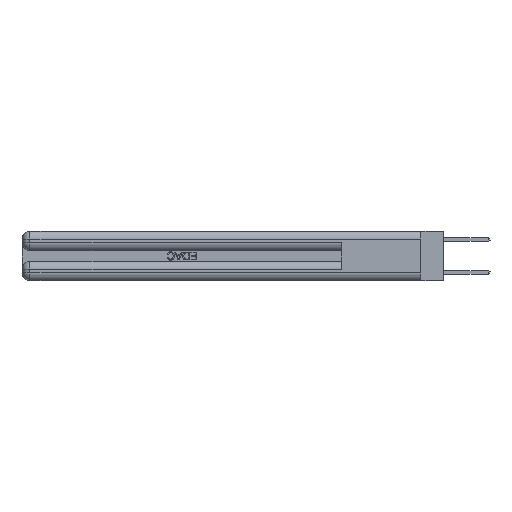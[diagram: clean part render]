
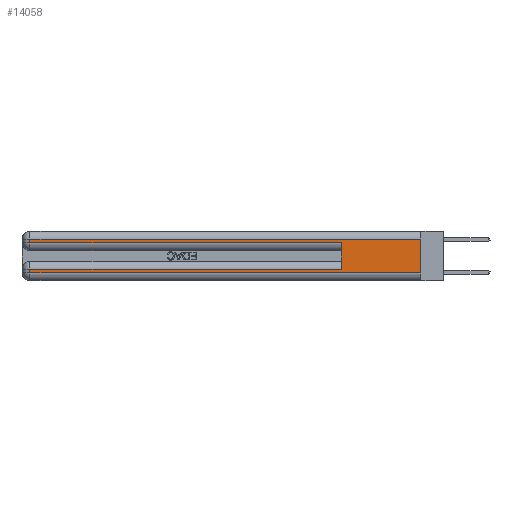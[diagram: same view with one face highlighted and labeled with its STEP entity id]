
A CAD part, left-side view. The second image highlights one B-rep face of the part: STEP entity #14058.
In plain terms, the highlighted planar face has unit normal (-1, 0, 0).
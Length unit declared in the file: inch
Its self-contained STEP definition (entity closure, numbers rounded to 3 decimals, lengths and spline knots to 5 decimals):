
#309 = VECTOR ( 'NONE', #28765, 39.37008 ) ;
#1189 = EDGE_CURVE ( 'NONE', #12646, #17756, #11935, .T. ) ;
#1290 = VECTOR ( 'NONE', #28421, 39.37008 ) ;
#1378 = LINE ( 'NONE', #26140, #14333 ) ;
#1954 = CARTESIAN_POINT ( 'NONE',  ( 0., 0., 0.06 ) ) ;
#2034 = DIRECTION ( 'NONE',  ( 0., 1., 0. ) ) ;
#3060 = DIRECTION ( 'NONE',  ( 0., 0., -1. ) ) ;
#3220 = VERTEX_POINT ( 'NONE', #25438 ) ;
#4101 = ORIENTED_EDGE ( 'NONE', *, *, #23650, .T. ) ;
#4545 = DIRECTION ( 'NONE',  ( 0., -1., 0. ) ) ;
#4770 = VECTOR ( 'NONE', #29475, 39.37008 ) ;
#5041 = VECTOR ( 'NONE', #29086, 39.37008 ) ;
#5283 = EDGE_LOOP ( 'NONE', ( #7089, #4101, #10918, #25118, #6736, #8065, #23968, #16320 ) ) ;
#6498 = LINE ( 'NONE', #11570, #12587 ) ;
#6736 = ORIENTED_EDGE ( 'NONE', *, *, #1189, .F. ) ;
#7089 = ORIENTED_EDGE ( 'NONE', *, *, #25392, .F. ) ;
#8065 = ORIENTED_EDGE ( 'NONE', *, *, #8126, .T. ) ;
#8126 = EDGE_CURVE ( 'NONE', #12646, #19858, #32157, .T. ) ;
#8192 = CARTESIAN_POINT ( 'NONE',  ( 0., 2.94, 0.37 ) ) ;
#8546 = AXIS2_PLACEMENT_3D ( 'NONE', #15978, #18500, #3060 ) ;
#10476 = CARTESIAN_POINT ( 'NONE',  ( 0., 0., 0.31 ) ) ;
#10918 = ORIENTED_EDGE ( 'NONE', *, *, #13367, .T. ) ;
#11570 = CARTESIAN_POINT ( 'NONE',  ( 0., 0., 0.37 ) ) ;
#11935 = LINE ( 'NONE', #18733, #5041 ) ;
#12197 = CARTESIAN_POINT ( 'NONE',  ( 0., 2.94, 0.06 ) ) ;
#12587 = VECTOR ( 'NONE', #20581, 39.37008 ) ;
#12646 = VERTEX_POINT ( 'NONE', #30498 ) ;
#12924 = EDGE_CURVE ( 'NONE', #19858, #27780, #31333, .T. ) ;
#13351 = VECTOR ( 'NONE', #2034, 39.37008 ) ;
#13367 = EDGE_CURVE ( 'NONE', #3220, #16617, #27677, .T. ) ;
#13630 = FACE_OUTER_BOUND ( 'NONE', #5283, .T. ) ;
#14058 = ADVANCED_FACE ( 'NONE', ( #13630 ), #31313, .F. ) ;
#14333 = VECTOR ( 'NONE', #31314, 39.37008 ) ;
#14904 = VECTOR ( 'NONE', #4545, 39.37008 ) ;
#15214 = VERTEX_POINT ( 'NONE', #23761 ) ;
#15978 = CARTESIAN_POINT ( 'NONE',  ( 0., 0., 0.37 ) ) ;
#16320 = ORIENTED_EDGE ( 'NONE', *, *, #18050, .T. ) ;
#16487 = LINE ( 'NONE', #1954, #14904 ) ;
#16617 = VERTEX_POINT ( 'NONE', #18949 ) ;
#16696 = CARTESIAN_POINT ( 'NONE',  ( 0., 2.94, 0.37 ) ) ;
#17510 = CARTESIAN_POINT ( 'NONE',  ( 0., 0., 0.085 ) ) ;
#17756 = VERTEX_POINT ( 'NONE', #24029 ) ;
#18050 = EDGE_CURVE ( 'NONE', #27780, #18763, #16487, .T. ) ;
#18500 = DIRECTION ( 'NONE',  ( 1., 0., 0. ) ) ;
#18733 = CARTESIAN_POINT ( 'NONE',  ( 0., 0.6, 0.145 ) ) ;
#18763 = VERTEX_POINT ( 'NONE', #30499 ) ;
#18949 = CARTESIAN_POINT ( 'NONE',  ( 0., 2.94, 0.285 ) ) ;
#19399 = CARTESIAN_POINT ( 'NONE',  ( 0., 2.94, 0.085 ) ) ;
#19858 = VERTEX_POINT ( 'NONE', #19399 ) ;
#20199 = EDGE_CURVE ( 'NONE', #16617, #17756, #1378, .T. ) ;
#20581 = DIRECTION ( 'NONE',  ( 0., 0., -1. ) ) ;
#21035 = LINE ( 'NONE', #10476, #1290 ) ;
#23650 = EDGE_CURVE ( 'NONE', #15214, #3220, #21035, .T. ) ;
#23761 = CARTESIAN_POINT ( 'NONE',  ( 0., 0., 0.31 ) ) ;
#23968 = ORIENTED_EDGE ( 'NONE', *, *, #12924, .T. ) ;
#24029 = CARTESIAN_POINT ( 'NONE',  ( 0., 0.6, 0.285 ) ) ;
#25118 = ORIENTED_EDGE ( 'NONE', *, *, #20199, .T. ) ;
#25392 = EDGE_CURVE ( 'NONE', #15214, #18763, #6498, .T. ) ;
#25438 = CARTESIAN_POINT ( 'NONE',  ( 0., 2.94, 0.31 ) ) ;
#26140 = CARTESIAN_POINT ( 'NONE',  ( 0., 0., 0.285 ) ) ;
#27677 = LINE ( 'NONE', #8192, #309 ) ;
#27780 = VERTEX_POINT ( 'NONE', #12197 ) ;
#28421 = DIRECTION ( 'NONE',  ( 0., 1., 0. ) ) ;
#28765 = DIRECTION ( 'NONE',  ( 0., 0., -1. ) ) ;
#29086 = DIRECTION ( 'NONE',  ( 0., 0., 1. ) ) ;
#29475 = DIRECTION ( 'NONE',  ( 0., 0., -1. ) ) ;
#30498 = CARTESIAN_POINT ( 'NONE',  ( 0., 0.6, 0.085 ) ) ;
#30499 = CARTESIAN_POINT ( 'NONE',  ( 0., 0., 0.06 ) ) ;
#31313 = PLANE ( 'NONE',  #8546 ) ;
#31314 = DIRECTION ( 'NONE',  ( 0., -1., 0. ) ) ;
#31333 = LINE ( 'NONE', #16696, #4770 ) ;
#32157 = LINE ( 'NONE', #17510, #13351 ) ;
